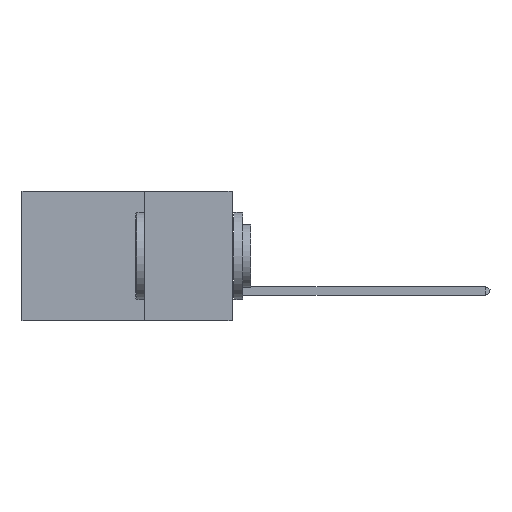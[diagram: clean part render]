
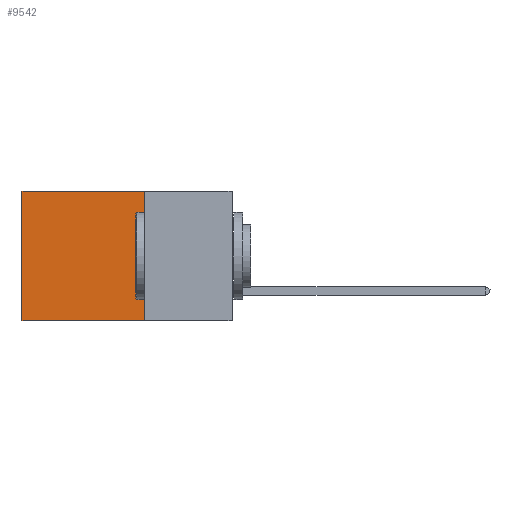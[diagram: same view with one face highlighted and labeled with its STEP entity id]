
A CAD part, left-side view. The second image highlights one B-rep face of the part: STEP entity #9542.
In plain terms, the highlighted planar face has unit normal (-1, 0, 0).
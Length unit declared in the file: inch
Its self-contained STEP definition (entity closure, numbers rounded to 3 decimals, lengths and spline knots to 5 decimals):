
#486 = FACE_OUTER_BOUND ( 'NONE', #13228, .T. ) ;
#1066 = DIRECTION ( 'NONE',  ( 0., 1., 0. ) ) ;
#1157 = CARTESIAN_POINT ( 'NONE',  ( 0.2875, 0.25, -0.37 ) ) ;
#1166 = EDGE_CURVE ( 'NONE', #7723, #4323, #13949, .T. ) ;
#1364 = DIRECTION ( 'NONE',  ( 0., 1., 0. ) ) ;
#1379 = LINE ( 'NONE', #11165, #12684 ) ;
#1767 = CARTESIAN_POINT ( 'NONE',  ( 0.2875, 0.25, 0. ) ) ;
#2132 = CARTESIAN_POINT ( 'NONE',  ( 0.2875, 0.25, 0. ) ) ;
#2419 = VERTEX_POINT ( 'NONE', #3715 ) ;
#2987 = CARTESIAN_POINT ( 'NONE',  ( 0.2875, 0.6, 0. ) ) ;
#3296 = PLANE ( 'NONE',  #10350 ) ;
#3715 = CARTESIAN_POINT ( 'NONE',  ( 0.2875, 0.25, -0.37 ) ) ;
#4323 = VERTEX_POINT ( 'NONE', #5572 ) ;
#5451 = ORIENTED_EDGE ( 'NONE', *, *, #1166, .T. ) ;
#5572 = CARTESIAN_POINT ( 'NONE',  ( 0.2875, 0.6, -0.37 ) ) ;
#6933 = VECTOR ( 'NONE', #1066, 39.37008 ) ;
#6990 = DIRECTION ( 'NONE',  ( 1., 0., 0. ) ) ;
#7321 = DIRECTION ( 'NONE',  ( 0., 0., -1. ) ) ;
#7608 = VECTOR ( 'NONE', #10158, 39.37008 ) ;
#7723 = VERTEX_POINT ( 'NONE', #7953 ) ;
#7953 = CARTESIAN_POINT ( 'NONE',  ( 0.2875, 0.6, 0. ) ) ;
#8663 = ORIENTED_EDGE ( 'NONE', *, *, #14103, .F. ) ;
#9110 = ORIENTED_EDGE ( 'NONE', *, *, #13531, .F. ) ;
#9542 = ADVANCED_FACE ( 'NONE', ( #486 ), #3296, .F. ) ;
#10158 = DIRECTION ( 'NONE',  ( 0., 0., -1. ) ) ;
#10350 = AXIS2_PLACEMENT_3D ( 'NONE', #2132, #6990, #12838 ) ;
#10742 = LINE ( 'NONE', #1157, #13145 ) ;
#11165 = CARTESIAN_POINT ( 'NONE',  ( 0.2875, 0.25, 0. ) ) ;
#11828 = CARTESIAN_POINT ( 'NONE',  ( 0.2875, 0.25, 0. ) ) ;
#11906 = VERTEX_POINT ( 'NONE', #1767 ) ;
#12684 = VECTOR ( 'NONE', #7321, 39.37008 ) ;
#12838 = DIRECTION ( 'NONE',  ( 0., 0., -1. ) ) ;
#13145 = VECTOR ( 'NONE', #1364, 39.37008 ) ;
#13228 = EDGE_LOOP ( 'NONE', ( #5451, #8663, #9110, #14158 ) ) ;
#13414 = EDGE_CURVE ( 'NONE', #11906, #7723, #15580, .T. ) ;
#13531 = EDGE_CURVE ( 'NONE', #11906, #2419, #1379, .T. ) ;
#13949 = LINE ( 'NONE', #2987, #7608 ) ;
#14103 = EDGE_CURVE ( 'NONE', #2419, #4323, #10742, .T. ) ;
#14158 = ORIENTED_EDGE ( 'NONE', *, *, #13414, .T. ) ;
#15580 = LINE ( 'NONE', #11828, #6933 ) ;
